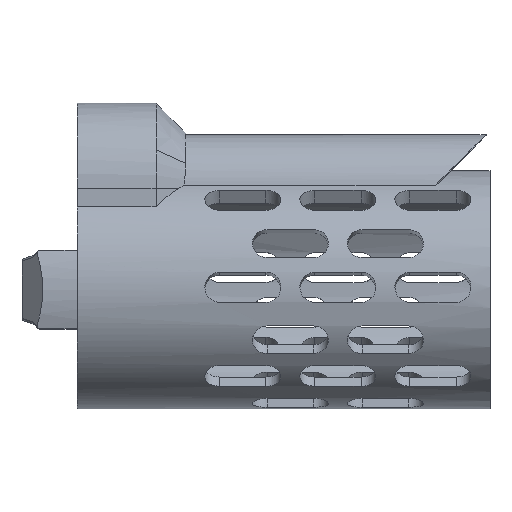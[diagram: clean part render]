
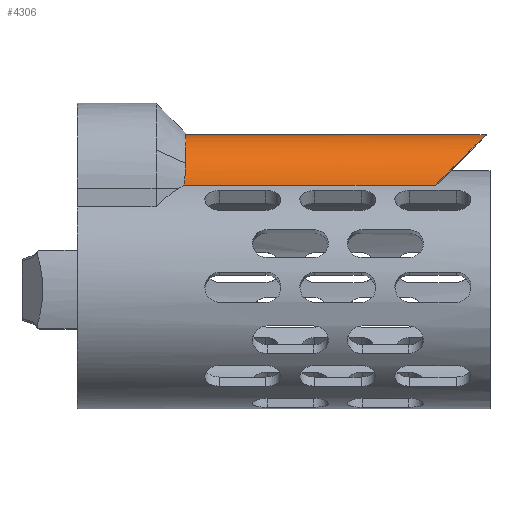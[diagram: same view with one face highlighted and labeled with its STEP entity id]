
A CAD part, top view. The second image highlights one B-rep face of the part: STEP entity #4306.
In plain terms, the highlighted cylindrical face has radius 13.5 mm (diameter 27 mm), a partial arc.
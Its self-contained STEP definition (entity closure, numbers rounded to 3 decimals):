
#131=CIRCLE('',#4579,13.5);
#208=CYLINDRICAL_SURFACE('',#4592,13.5);
#301=LINE('',#6046,#672);
#305=LINE('',#6070,#676);
#375=LINE('',#7439,#746);
#672=VECTOR('',#4866,10.);
#676=VECTOR('',#4884,10.);
#746=VECTOR('',#4984,10.);
#1208=FACE_OUTER_BOUND('',#1498,.T.);
#1498=EDGE_LOOP('',(#3413,#3414,#3415,#3416,#3417,#3418,#3419,#3420,#3421,
#3422));
#1704=B_SPLINE_CURVE_WITH_KNOTS('',3,(#6022,#6023,#6024,#6025,#6026,#6027,
#6028,#6029,#6030,#6031),.UNSPECIFIED.,.F.,.F.,(4,1,1,1,1,1,1,4),(-1.077,
-0.723,-0.359,0.005,0.368,
0.732,1.096,1.459),.UNSPECIFIED.);
#1768=B_SPLINE_CURVE_WITH_KNOTS('',3,(#7341,#7342,#7343,#7344,#7345,#7346,
#7347),.UNSPECIFIED.,.F.,.F.,(4,3,4),(0.,0.016,0.033),
 .UNSPECIFIED.);
#1772=B_SPLINE_CURVE_WITH_KNOTS('',3,(#7369,#7370,#7371,#7372),
 .UNSPECIFIED.,.F.,.F.,(4,4),(1.405,1.426),
 .UNSPECIFIED.);
#1773=B_SPLINE_CURVE_WITH_KNOTS('',3,(#7373,#7374,#7375,#7376),
 .UNSPECIFIED.,.F.,.F.,(4,4),(0.551,0.57),
 .UNSPECIFIED.);
#1779=B_SPLINE_CURVE_WITH_KNOTS('',3,(#7447,#7448,#7449,#7450),
 .UNSPECIFIED.,.F.,.F.,(4,4),(4.793,4.838),
 .UNSPECIFIED.);
#1780=B_SPLINE_CURVE_WITH_KNOTS('',3,(#7467,#7468,#7469,#7470,#7471,#7472),
 .UNSPECIFIED.,.F.,.F.,(4,2,4),(0.,0.535,0.545),
 .UNSPECIFIED.);
#1874=VERTEX_POINT('',#6016);
#1875=VERTEX_POINT('',#6021);
#1877=VERTEX_POINT('',#6042);
#1882=VERTEX_POINT('',#6069);
#2007=VERTEX_POINT('',#7332);
#2008=VERTEX_POINT('',#7340);
#2011=VERTEX_POINT('',#7368);
#2023=VERTEX_POINT('',#7429);
#2025=VERTEX_POINT('',#7443);
#2026=VERTEX_POINT('',#7445);
#2301=EDGE_CURVE('',#1874,#1875,#1704,.T.);
#2305=EDGE_CURVE('',#1877,#1874,#301,.T.);
#2313=EDGE_CURVE('',#1875,#1882,#305,.T.);
#2441=EDGE_CURVE('',#2008,#2007,#1768,.T.);
#2445=EDGE_CURVE('',#2011,#2008,#1772,.T.);
#2446=EDGE_CURVE('',#2011,#1877,#1773,.T.);
#2464=EDGE_CURVE('',#2023,#2007,#375,.T.);
#2468=EDGE_CURVE('',#2026,#2023,#1779,.F.);
#2469=EDGE_CURVE('',#2025,#1882,#1780,.T.);
#2652=EDGE_CURVE('',#2025,#2026,#131,.T.);
#3413=ORIENTED_EDGE('',*,*,#2446,.F.);
#3414=ORIENTED_EDGE('',*,*,#2445,.T.);
#3415=ORIENTED_EDGE('',*,*,#2441,.T.);
#3416=ORIENTED_EDGE('',*,*,#2464,.F.);
#3417=ORIENTED_EDGE('',*,*,#2468,.F.);
#3418=ORIENTED_EDGE('',*,*,#2652,.F.);
#3419=ORIENTED_EDGE('',*,*,#2469,.T.);
#3420=ORIENTED_EDGE('',*,*,#2313,.F.);
#3421=ORIENTED_EDGE('',*,*,#2301,.F.);
#3422=ORIENTED_EDGE('',*,*,#2305,.F.);
#4306=ADVANCED_FACE('',(#1208),#208,.T.);
#4579=AXIS2_PLACEMENT_3D('',#8867,#5158,#5159);
#4592=AXIS2_PLACEMENT_3D('',#8891,#5191,#5192);
#4866=DIRECTION('',(1.,0.,0.));
#4884=DIRECTION('',(-1.,0.,0.));
#4984=DIRECTION('',(1.,0.,0.));
#5158=DIRECTION('center_axis',(-1.,0.,0.));
#5159=DIRECTION('ref_axis',(0.,1.,0.));
#5191=DIRECTION('center_axis',(1.,0.,0.));
#5192=DIRECTION('ref_axis',(0.,1.,0.));
#6016=CARTESIAN_POINT('',(100.714,53.03,-10.827));
#6021=CARTESIAN_POINT('',(95.831,48.164,14.4));
#6022=CARTESIAN_POINT('Ctrl Pts',(100.714,53.03,-10.827));
#6023=CARTESIAN_POINT('Ctrl Pts',(102.116,54.425,-10.059));
#6024=CARTESIAN_POINT('Ctrl Pts',(104.677,56.967,-8.003));
#6025=CARTESIAN_POINT('Ctrl Pts',(107.202,59.462,-3.778));
#6026=CARTESIAN_POINT('Ctrl Pts',(108.066,60.312,1.063));
#6027=CARTESIAN_POINT('Ctrl Pts',(107.157,59.417,5.897));
#6028=CARTESIAN_POINT('Ctrl Pts',(104.572,56.863,10.134));
#6029=CARTESIAN_POINT('Ctrl Pts',(100.636,52.957,13.206));
#6030=CARTESIAN_POINT('Ctrl Pts',(97.457,49.787,14.201));
#6031=CARTESIAN_POINT('Ctrl Pts',(95.831,48.164,14.4));
#6042=CARTESIAN_POINT('',(95.284,53.03,-10.827));
#6046=CARTESIAN_POINT('',(88.7,53.03,-10.827));
#6069=CARTESIAN_POINT('',(36.865,48.164,14.4));
#6070=CARTESIAN_POINT('',(37.189,48.164,14.4));
#7332=CARTESIAN_POINT('',(95.018,52.855,-10.922));
#7340=CARTESIAN_POINT('',(95.261,52.659,-11.024));
#7341=CARTESIAN_POINT('Ctrl Pts',(95.261,52.659,-11.024));
#7342=CARTESIAN_POINT('Ctrl Pts',(95.22,52.692,-11.007));
#7343=CARTESIAN_POINT('Ctrl Pts',(95.18,52.725,-10.99));
#7344=CARTESIAN_POINT('Ctrl Pts',(95.14,52.757,-10.974));
#7345=CARTESIAN_POINT('Ctrl Pts',(95.099,52.79,-10.957));
#7346=CARTESIAN_POINT('Ctrl Pts',(95.058,52.823,-10.94));
#7347=CARTESIAN_POINT('Ctrl Pts',(95.017,52.855,-10.922));
#7368=CARTESIAN_POINT('',(95.273,52.855,-10.922));
#7369=CARTESIAN_POINT('Ctrl Pts',(95.273,52.855,-10.922));
#7370=CARTESIAN_POINT('Ctrl Pts',(95.269,52.79,-10.957));
#7371=CARTESIAN_POINT('Ctrl Pts',(95.265,52.725,-10.99));
#7372=CARTESIAN_POINT('Ctrl Pts',(95.261,52.659,-11.024));
#7373=CARTESIAN_POINT('Ctrl Pts',(95.273,52.855,-10.922));
#7374=CARTESIAN_POINT('Ctrl Pts',(95.277,52.913,-10.891));
#7375=CARTESIAN_POINT('Ctrl Pts',(95.281,52.972,-10.859));
#7376=CARTESIAN_POINT('Ctrl Pts',(95.284,53.03,-10.827));
#7429=CARTESIAN_POINT('',(37.162,52.855,-10.922));
#7439=CARTESIAN_POINT('',(37.189,52.855,-10.922));
#7443=CARTESIAN_POINT('',(37.189,53.272,12.691));
#7445=CARTESIAN_POINT('',(37.189,53.272,-10.691));
#7447=CARTESIAN_POINT('Ctrl Pts',(37.162,52.855,-10.922));
#7448=CARTESIAN_POINT('Ctrl Pts',(37.171,52.995,-10.848));
#7449=CARTESIAN_POINT('Ctrl Pts',(37.18,53.134,-10.77));
#7450=CARTESIAN_POINT('Ctrl Pts',(37.189,53.272,-10.691));
#7467=CARTESIAN_POINT('Ctrl Pts',(37.189,53.272,12.691));
#7468=CARTESIAN_POINT('Ctrl Pts',(37.09,51.73,13.581));
#7469=CARTESIAN_POINT('Ctrl Pts',(36.982,50.028,14.157));
#7470=CARTESIAN_POINT('Ctrl Pts',(36.869,48.23,14.391));
#7471=CARTESIAN_POINT('Ctrl Pts',(36.867,48.197,14.396));
#7472=CARTESIAN_POINT('Ctrl Pts',(36.865,48.164,14.4));
#8867=CARTESIAN_POINT('Origin',(37.189,46.521,1.));
#8891=CARTESIAN_POINT('Origin',(37.189,46.521,1.));
